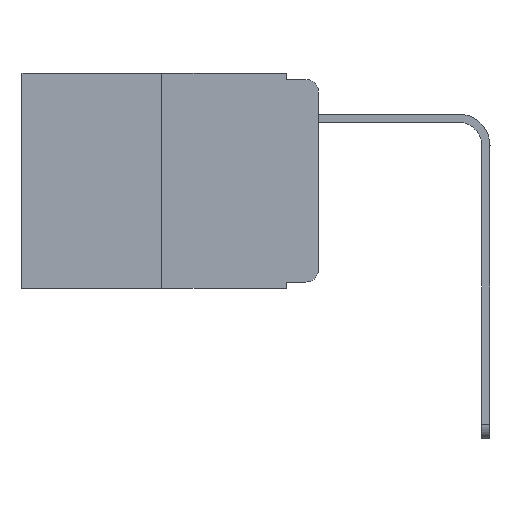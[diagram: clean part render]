
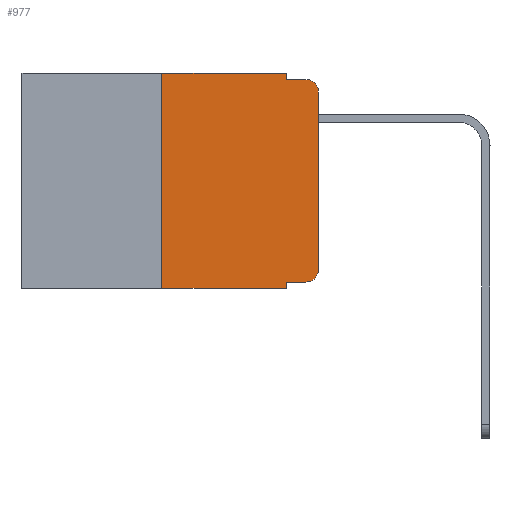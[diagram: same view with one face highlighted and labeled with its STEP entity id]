
A CAD part, left-side view. The second image highlights one B-rep face of the part: STEP entity #977.
In plain terms, the highlighted planar face has unit normal (-1, 0, 0).
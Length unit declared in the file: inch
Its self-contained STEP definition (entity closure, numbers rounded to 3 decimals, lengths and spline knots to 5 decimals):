
#81 = PLANE ( 'NONE',  #15486 ) ;
#166 = VECTOR ( 'NONE', #3060, 39.37008 ) ;
#340 = LINE ( 'NONE', #8186, #10107 ) ;
#580 = ORIENTED_EDGE ( 'NONE', *, *, #1524, .T. ) ;
#679 = VERTEX_POINT ( 'NONE', #9427 ) ;
#977 = ADVANCED_FACE ( 'NONE', ( #14397 ), #81, .F. ) ;
#1155 = ORIENTED_EDGE ( 'NONE', *, *, #16522, .T. ) ;
#1524 = EDGE_CURVE ( 'NONE', #679, #16535, #5348, .T. ) ;
#1574 = CARTESIAN_POINT ( 'NONE',  ( 0., 0.473, 0. ) ) ;
#1616 = VERTEX_POINT ( 'NONE', #5081 ) ;
#2339 = DIRECTION ( 'NONE',  ( -1., 0., 0. ) ) ;
#2586 = AXIS2_PLACEMENT_3D ( 'NONE', #12188, #16612, #4702 ) ;
#3060 = DIRECTION ( 'NONE',  ( 0., -1., 0. ) ) ;
#3109 = VERTEX_POINT ( 'NONE', #14302 ) ;
#3292 = VERTEX_POINT ( 'NONE', #6375 ) ;
#3305 = CIRCLE ( 'NONE', #4541, 0.02 ) ;
#3350 = ORIENTED_EDGE ( 'NONE', *, *, #14576, .T. ) ;
#3396 = VERTEX_POINT ( 'NONE', #17256 ) ;
#3733 = EDGE_CURVE ( 'NONE', #16857, #3396, #8022, .T. ) ;
#3851 = CARTESIAN_POINT ( 'NONE',  ( 0., 0.473, 0. ) ) ;
#3992 = ORIENTED_EDGE ( 'NONE', *, *, #11733, .T. ) ;
#4541 = AXIS2_PLACEMENT_3D ( 'NONE', #17145, #2339, #6647 ) ;
#4567 = VERTEX_POINT ( 'NONE', #10704 ) ;
#4579 = DIRECTION ( 'NONE',  ( 0., -1., 0. ) ) ;
#4702 = DIRECTION ( 'NONE',  ( 0., 0., -1. ) ) ;
#4705 = CARTESIAN_POINT ( 'NONE',  ( 0., 0.473, -0.343 ) ) ;
#4786 = DIRECTION ( 'NONE',  ( 0., 0., -1. ) ) ;
#4917 = EDGE_CURVE ( 'NONE', #4567, #17532, #14253, .T. ) ;
#5081 = CARTESIAN_POINT ( 'NONE',  ( 0., 0.051, -0.333 ) ) ;
#5258 = VERTEX_POINT ( 'NONE', #5993 ) ;
#5348 = CIRCLE ( 'NONE', #2586, 0.02 ) ;
#5993 = CARTESIAN_POINT ( 'NONE',  ( 0., 0.051, -0.343 ) ) ;
#5997 = VECTOR ( 'NONE', #19028, 39.37008 ) ;
#6375 = CARTESIAN_POINT ( 'NONE',  ( 0., 0.25, -0.343 ) ) ;
#6390 = VECTOR ( 'NONE', #18840, 39.37008 ) ;
#6622 = EDGE_CURVE ( 'NONE', #3109, #3396, #3305, .T. ) ;
#6647 = DIRECTION ( 'NONE',  ( 0., 0., -1. ) ) ;
#7154 = VECTOR ( 'NONE', #16350, 39.37008 ) ;
#7220 = ORIENTED_EDGE ( 'NONE', *, *, #14336, .F. ) ;
#7363 = ORIENTED_EDGE ( 'NONE', *, *, #15879, .F. ) ;
#7408 = CARTESIAN_POINT ( 'NONE',  ( 0., 0.25, 0. ) ) ;
#7664 = DIRECTION ( 'NONE',  ( 1., 0., 0. ) ) ;
#7712 = CARTESIAN_POINT ( 'NONE',  ( 0., 0.051, -0.333 ) ) ;
#8022 = LINE ( 'NONE', #9014, #166 ) ;
#8186 = CARTESIAN_POINT ( 'NONE',  ( 0., 0.051, 0. ) ) ;
#9014 = CARTESIAN_POINT ( 'NONE',  ( 0., 0.051, -0.01 ) ) ;
#9427 = CARTESIAN_POINT ( 'NONE',  ( 0., 0.02, -0.333 ) ) ;
#9637 = DIRECTION ( 'NONE',  ( 0., 0., -1. ) ) ;
#10107 = VECTOR ( 'NONE', #9637, 39.37008 ) ;
#10704 = CARTESIAN_POINT ( 'NONE',  ( 0., 0.25, 0. ) ) ;
#10921 = LINE ( 'NONE', #4705, #16251 ) ;
#11199 = ORIENTED_EDGE ( 'NONE', *, *, #6622, .T. ) ;
#11547 = LINE ( 'NONE', #7712, #16177 ) ;
#11733 = EDGE_CURVE ( 'NONE', #1616, #679, #11547, .T. ) ;
#12188 = CARTESIAN_POINT ( 'NONE',  ( 0., 0.02, -0.313 ) ) ;
#12626 = DIRECTION ( 'NONE',  ( 0., -1., 0. ) ) ;
#12936 = LINE ( 'NONE', #14609, #5997 ) ;
#13114 = CARTESIAN_POINT ( 'NONE',  ( 0., 0., 0. ) ) ;
#13374 = VECTOR ( 'NONE', #17421, 39.37008 ) ;
#13547 = EDGE_LOOP ( 'NONE', ( #1155, #11199, #15949, #18525, #16180, #7220, #3350, #7363, #3992, #580 ) ) ;
#14253 = LINE ( 'NONE', #3851, #6390 ) ;
#14302 = CARTESIAN_POINT ( 'NONE',  ( 0., 0., -0.03 ) ) ;
#14336 = EDGE_CURVE ( 'NONE', #3292, #4567, #15269, .T. ) ;
#14397 = FACE_OUTER_BOUND ( 'NONE', #13547, .T. ) ;
#14576 = EDGE_CURVE ( 'NONE', #3292, #5258, #10921, .T. ) ;
#14609 = CARTESIAN_POINT ( 'NONE',  ( 0., 0.051, 0. ) ) ;
#15269 = LINE ( 'NONE', #7408, #7154 ) ;
#15486 = AXIS2_PLACEMENT_3D ( 'NONE', #1574, #7664, #4786 ) ;
#15487 = CARTESIAN_POINT ( 'NONE',  ( 0., 0.051, -0.01 ) ) ;
#15532 = CARTESIAN_POINT ( 'NONE',  ( 0., 0.051, 0. ) ) ;
#15879 = EDGE_CURVE ( 'NONE', #1616, #5258, #12936, .T. ) ;
#15914 = CARTESIAN_POINT ( 'NONE',  ( 0., 0., -0.313 ) ) ;
#15949 = ORIENTED_EDGE ( 'NONE', *, *, #3733, .F. ) ;
#16177 = VECTOR ( 'NONE', #4579, 39.37008 ) ;
#16180 = ORIENTED_EDGE ( 'NONE', *, *, #4917, .F. ) ;
#16251 = VECTOR ( 'NONE', #12626, 39.37008 ) ;
#16350 = DIRECTION ( 'NONE',  ( 0., 0., 1. ) ) ;
#16522 = EDGE_CURVE ( 'NONE', #16535, #3109, #17328, .T. ) ;
#16535 = VERTEX_POINT ( 'NONE', #15914 ) ;
#16612 = DIRECTION ( 'NONE',  ( -1., 0., 0. ) ) ;
#16857 = VERTEX_POINT ( 'NONE', #15487 ) ;
#17145 = CARTESIAN_POINT ( 'NONE',  ( 0., 0.02, -0.03 ) ) ;
#17256 = CARTESIAN_POINT ( 'NONE',  ( 0., 0.02, -0.01 ) ) ;
#17328 = LINE ( 'NONE', #13114, #13374 ) ;
#17421 = DIRECTION ( 'NONE',  ( 0., 0., 1. ) ) ;
#17455 = EDGE_CURVE ( 'NONE', #17532, #16857, #340, .T. ) ;
#17532 = VERTEX_POINT ( 'NONE', #15532 ) ;
#18525 = ORIENTED_EDGE ( 'NONE', *, *, #17455, .F. ) ;
#18840 = DIRECTION ( 'NONE',  ( 0., -1., 0. ) ) ;
#19028 = DIRECTION ( 'NONE',  ( 0., 0., -1. ) ) ;
